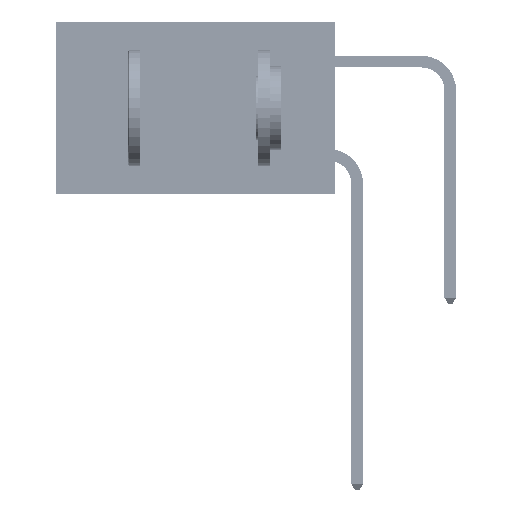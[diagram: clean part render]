
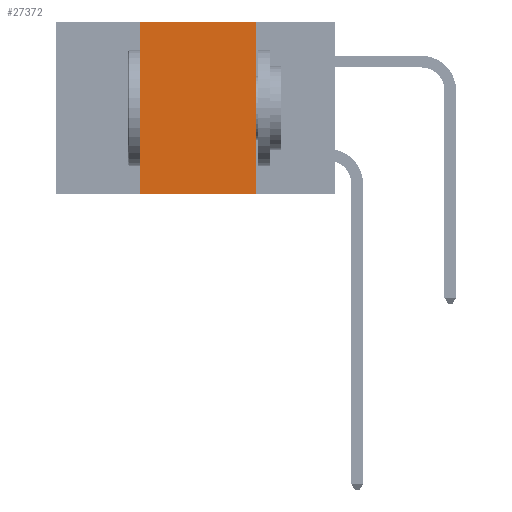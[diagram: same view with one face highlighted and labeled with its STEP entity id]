
A CAD part, left-side view. The second image highlights one B-rep face of the part: STEP entity #27372.
In plain terms, the highlighted planar face has unit normal (-1, 0, 0).
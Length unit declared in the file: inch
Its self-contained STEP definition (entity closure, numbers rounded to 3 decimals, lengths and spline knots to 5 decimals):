
#1150 = CARTESIAN_POINT ( 'NONE',  ( 0., 0.17, -0.37 ) ) ;
#1215 = CARTESIAN_POINT ( 'NONE',  ( 0., 0.6, 0. ) ) ;
#2189 = VECTOR ( 'NONE', #23658, 39.37008 ) ;
#2298 = EDGE_CURVE ( 'NONE', #45242, #15750, #52124, .T. ) ;
#2488 = CARTESIAN_POINT ( 'NONE',  ( 0., 0.6, -0.37 ) ) ;
#5854 = VECTOR ( 'NONE', #17253, 39.37008 ) ;
#6780 = CARTESIAN_POINT ( 'NONE',  ( 0., 0.6, 0. ) ) ;
#9248 = CARTESIAN_POINT ( 'NONE',  ( 0., 0.42, 0. ) ) ;
#11337 = CARTESIAN_POINT ( 'NONE',  ( 0., 0.42, -0.37 ) ) ;
#13084 = CARTESIAN_POINT ( 'NONE',  ( 0., 0.42, 0. ) ) ;
#15750 = VERTEX_POINT ( 'NONE', #1150 ) ;
#16045 = AXIS2_PLACEMENT_3D ( 'NONE', #1215, #46309, #42131 ) ;
#16346 = ORIENTED_EDGE ( 'NONE', *, *, #2298, .T. ) ;
#17253 = DIRECTION ( 'NONE',  ( 0., 0., 1. ) ) ;
#22893 = ORIENTED_EDGE ( 'NONE', *, *, #43872, .F. ) ;
#23601 = DIRECTION ( 'NONE',  ( 0., 0., -1. ) ) ;
#23658 = DIRECTION ( 'NONE',  ( 0., -1., 0. ) ) ;
#23762 = CARTESIAN_POINT ( 'NONE',  ( 0., 0.17, 0. ) ) ;
#25514 = LINE ( 'NONE', #6780, #2189 ) ;
#27372 = ADVANCED_FACE ( 'NONE', ( #50827 ), #38165, .F. ) ;
#27698 = EDGE_CURVE ( 'NONE', #31281, #30659, #25514, .T. ) ;
#30410 = ORIENTED_EDGE ( 'NONE', *, *, #50928, .F. ) ;
#30659 = VERTEX_POINT ( 'NONE', #33308 ) ;
#31281 = VERTEX_POINT ( 'NONE', #9248 ) ;
#33308 = CARTESIAN_POINT ( 'NONE',  ( 0., 0.17, 0. ) ) ;
#38165 = PLANE ( 'NONE',  #16045 ) ;
#39390 = VECTOR ( 'NONE', #23601, 39.37008 ) ;
#42131 = DIRECTION ( 'NONE',  ( 0., 0., -1. ) ) ;
#42612 = LINE ( 'NONE', #23762, #39390 ) ;
#43872 = EDGE_CURVE ( 'NONE', #30659, #15750, #42612, .T. ) ;
#44090 = LINE ( 'NONE', #13084, #5854 ) ;
#45242 = VERTEX_POINT ( 'NONE', #11337 ) ;
#46309 = DIRECTION ( 'NONE',  ( 1., 0., 0. ) ) ;
#48817 = DIRECTION ( 'NONE',  ( 0., -1., 0. ) ) ;
#50827 = FACE_OUTER_BOUND ( 'NONE', #51294, .T. ) ;
#50928 = EDGE_CURVE ( 'NONE', #45242, #31281, #44090, .T. ) ;
#51058 = ORIENTED_EDGE ( 'NONE', *, *, #27698, .F. ) ;
#51294 = EDGE_LOOP ( 'NONE', ( #22893, #51058, #30410, #16346 ) ) ;
#52124 = LINE ( 'NONE', #2488, #53419 ) ;
#53419 = VECTOR ( 'NONE', #48817, 39.37008 ) ;
